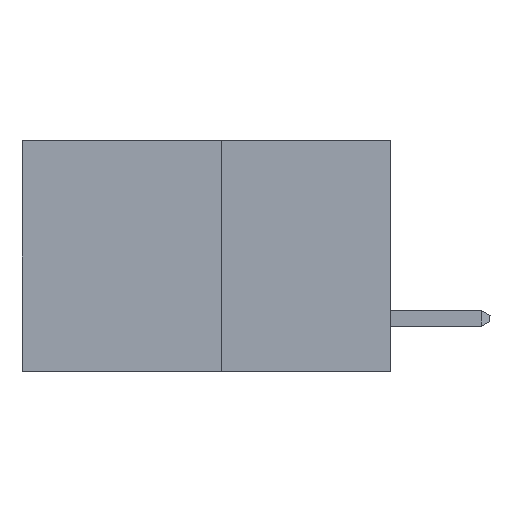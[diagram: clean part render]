
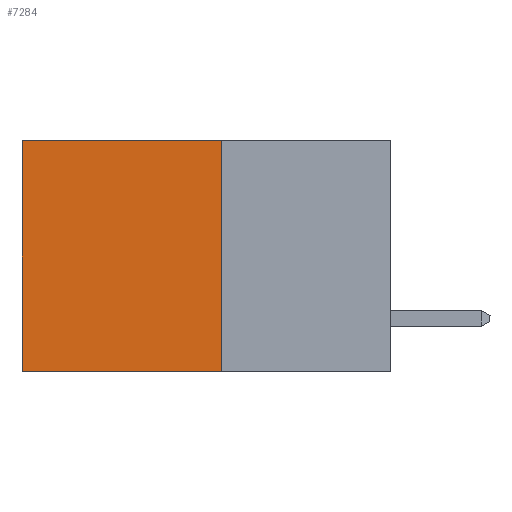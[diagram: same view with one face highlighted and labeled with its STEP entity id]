
A CAD part, left-side view. The second image highlights one B-rep face of the part: STEP entity #7284.
In plain terms, the highlighted planar face has unit normal (-1, 0, 0).
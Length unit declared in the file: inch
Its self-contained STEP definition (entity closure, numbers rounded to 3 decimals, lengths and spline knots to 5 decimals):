
#199 = CARTESIAN_POINT ( 'NONE',  ( 0.277, 0.27, -0.37 ) ) ;
#376 = EDGE_CURVE ( 'NONE', #4658, #9001, #11826, .T. ) ;
#655 = ORIENTED_EDGE ( 'NONE', *, *, #1081, .F. ) ;
#951 = LINE ( 'NONE', #199, #5828 ) ;
#1081 = EDGE_CURVE ( 'NONE', #2614, #9064, #951, .T. ) ;
#1368 = FACE_OUTER_BOUND ( 'NONE', #4152, .T. ) ;
#1489 = VECTOR ( 'NONE', #8333, 39.37008 ) ;
#2141 = ORIENTED_EDGE ( 'NONE', *, *, #8149, .F. ) ;
#2244 = DIRECTION ( 'NONE',  ( 0., 0., -1. ) ) ;
#2614 = VERTEX_POINT ( 'NONE', #7148 ) ;
#2633 = VECTOR ( 'NONE', #2244, 39.37008 ) ;
#2851 = CARTESIAN_POINT ( 'NONE',  ( 0.277, 0.27, -0.37 ) ) ;
#3338 = DIRECTION ( 'NONE',  ( 0., 1., 0. ) ) ;
#3549 = PLANE ( 'NONE',  #10195 ) ;
#3890 = LINE ( 'NONE', #2851, #1489 ) ;
#4152 = EDGE_LOOP ( 'NONE', ( #5995, #655, #2141, #6550 ) ) ;
#4300 = CARTESIAN_POINT ( 'NONE',  ( 0.277, 0.27, 0. ) ) ;
#4513 = CARTESIAN_POINT ( 'NONE',  ( 0.277, 0.27, -0.37 ) ) ;
#4658 = VERTEX_POINT ( 'NONE', #4300 ) ;
#5060 = LINE ( 'NONE', #5823, #2633 ) ;
#5436 = DIRECTION ( 'NONE',  ( 0., 0., -1. ) ) ;
#5823 = CARTESIAN_POINT ( 'NONE',  ( 0.277, 0.59, -0.37 ) ) ;
#5828 = VECTOR ( 'NONE', #6474, 39.37008 ) ;
#5995 = ORIENTED_EDGE ( 'NONE', *, *, #10326, .T. ) ;
#6124 = CARTESIAN_POINT ( 'NONE',  ( 0.277, 0.59, 0. ) ) ;
#6204 = CARTESIAN_POINT ( 'NONE',  ( 0.277, 0.59, -0.37 ) ) ;
#6474 = DIRECTION ( 'NONE',  ( 0., 1., 0. ) ) ;
#6550 = ORIENTED_EDGE ( 'NONE', *, *, #376, .T. ) ;
#7148 = CARTESIAN_POINT ( 'NONE',  ( 0.277, 0.27, -0.37 ) ) ;
#7284 = ADVANCED_FACE ( 'NONE', ( #1368 ), #3549, .F. ) ;
#8149 = EDGE_CURVE ( 'NONE', #4658, #2614, #3890, .T. ) ;
#8333 = DIRECTION ( 'NONE',  ( 0., 0., -1. ) ) ;
#9001 = VERTEX_POINT ( 'NONE', #6124 ) ;
#9064 = VERTEX_POINT ( 'NONE', #6204 ) ;
#10195 = AXIS2_PLACEMENT_3D ( 'NONE', #4513, #10763, #5436 ) ;
#10326 = EDGE_CURVE ( 'NONE', #9001, #9064, #5060, .T. ) ;
#10763 = DIRECTION ( 'NONE',  ( 1., 0., 0. ) ) ;
#11137 = CARTESIAN_POINT ( 'NONE',  ( 0.277, 0.27, 0. ) ) ;
#11296 = VECTOR ( 'NONE', #3338, 39.37008 ) ;
#11826 = LINE ( 'NONE', #11137, #11296 ) ;
